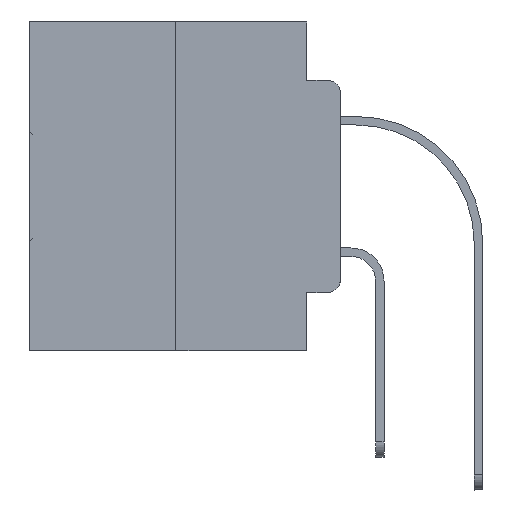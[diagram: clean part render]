
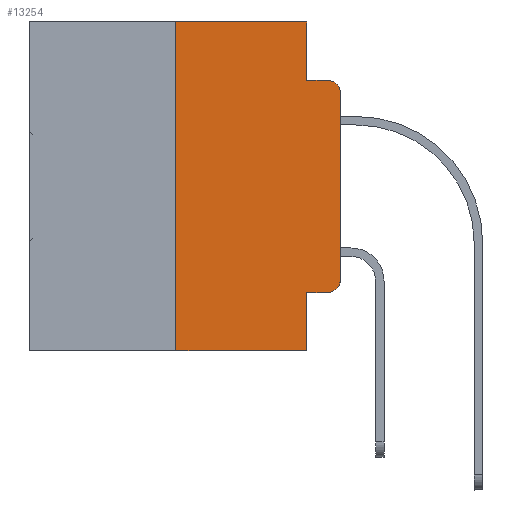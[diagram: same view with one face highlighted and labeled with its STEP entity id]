
A CAD part, left-side view. The second image highlights one B-rep face of the part: STEP entity #13254.
In plain terms, the highlighted planar face has unit normal (-1, 0, 0).
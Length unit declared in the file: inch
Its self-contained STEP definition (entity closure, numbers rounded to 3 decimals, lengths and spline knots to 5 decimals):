
#569 = VECTOR ( 'NONE', #16032, 39.37008 ) ;
#647 = DIRECTION ( 'NONE',  ( 0., -1., 0. ) ) ;
#1013 = ORIENTED_EDGE ( 'NONE', *, *, #14239, .T. ) ;
#1118 = DIRECTION ( 'NONE',  ( 0., 0., 1. ) ) ;
#1157 = DIRECTION ( 'NONE',  ( 0., 0., -1. ) ) ;
#1523 = ORIENTED_EDGE ( 'NONE', *, *, #28385, .T. ) ;
#1651 = CIRCLE ( 'NONE', #7608, 0.02 ) ;
#1792 = ORIENTED_EDGE ( 'NONE', *, *, #4485, .F. ) ;
#2020 = EDGE_CURVE ( 'NONE', #20331, #15721, #5002, .T. ) ;
#2157 = CARTESIAN_POINT ( 'NONE',  ( 0., 0.473, 0. ) ) ;
#2500 = VERTEX_POINT ( 'NONE', #3245 ) ;
#2501 = EDGE_LOOP ( 'NONE', ( #1523, #11395, #4385, #7156, #28050, #1792, #4592, #26779, #1013, #17779 ) ) ;
#2901 = VERTEX_POINT ( 'NONE', #24374 ) ;
#3165 = EDGE_CURVE ( 'NONE', #2500, #25275, #1651, .T. ) ;
#3245 = CARTESIAN_POINT ( 'NONE',  ( 0., 0., -0.1085 ) ) ;
#4208 = FACE_OUTER_BOUND ( 'NONE', #2501, .T. ) ;
#4333 = EDGE_CURVE ( 'NONE', #11425, #25275, #31983, .T. ) ;
#4385 = ORIENTED_EDGE ( 'NONE', *, *, #4333, .F. ) ;
#4485 = EDGE_CURVE ( 'NONE', #24267, #2901, #19437, .T. ) ;
#4533 = DIRECTION ( 'NONE',  ( -1., 0., 0. ) ) ;
#4592 = ORIENTED_EDGE ( 'NONE', *, *, #19235, .T. ) ;
#5002 = LINE ( 'NONE', #15340, #5952 ) ;
#5378 = CARTESIAN_POINT ( 'NONE',  ( 0., 0., -0.3915 ) ) ;
#5712 = LINE ( 'NONE', #31620, #569 ) ;
#5952 = VECTOR ( 'NONE', #25667, 39.37008 ) ;
#6264 = CARTESIAN_POINT ( 'NONE',  ( 0., 0.25, -0.5 ) ) ;
#6604 = AXIS2_PLACEMENT_3D ( 'NONE', #10593, #23294, #15172 ) ;
#6841 = VERTEX_POINT ( 'NONE', #17994 ) ;
#6898 = DIRECTION ( 'NONE',  ( 0., 0., -1. ) ) ;
#7156 = ORIENTED_EDGE ( 'NONE', *, *, #7508, .F. ) ;
#7508 = EDGE_CURVE ( 'NONE', #6841, #11425, #21168, .T. ) ;
#7608 = AXIS2_PLACEMENT_3D ( 'NONE', #19430, #4533, #6898 ) ;
#9150 = VERTEX_POINT ( 'NONE', #5378 ) ;
#9640 = DIRECTION ( 'NONE',  ( 0., 0., -1. ) ) ;
#9806 = PLANE ( 'NONE',  #13371 ) ;
#10593 = CARTESIAN_POINT ( 'NONE',  ( 0., 0.02, -0.3915 ) ) ;
#11395 = ORIENTED_EDGE ( 'NONE', *, *, #3165, .T. ) ;
#11425 = VERTEX_POINT ( 'NONE', #17455 ) ;
#11766 = LINE ( 'NONE', #22102, #21920 ) ;
#12451 = VECTOR ( 'NONE', #1118, 39.37008 ) ;
#12550 = CIRCLE ( 'NONE', #6604, 0.02 ) ;
#12561 = EDGE_CURVE ( 'NONE', #27626, #9150, #12550, .T. ) ;
#13227 = CARTESIAN_POINT ( 'NONE',  ( 0., 0.051, -0.5 ) ) ;
#13254 = ADVANCED_FACE ( 'NONE', ( #4208 ), #9806, .F. ) ;
#13371 = AXIS2_PLACEMENT_3D ( 'NONE', #2157, #29968, #9640 ) ;
#14180 = VECTOR ( 'NONE', #30111, 39.37008 ) ;
#14239 = EDGE_CURVE ( 'NONE', #20331, #27626, #17836, .T. ) ;
#14314 = CARTESIAN_POINT ( 'NONE',  ( 0., 0.02, -0.0885 ) ) ;
#15172 = DIRECTION ( 'NONE',  ( 0., 0., -1. ) ) ;
#15340 = CARTESIAN_POINT ( 'NONE',  ( 0., 0.051, 0. ) ) ;
#15721 = VERTEX_POINT ( 'NONE', #13227 ) ;
#16032 = DIRECTION ( 'NONE',  ( 0., -1., 0. ) ) ;
#17455 = CARTESIAN_POINT ( 'NONE',  ( 0., 0.051, -0.0885 ) ) ;
#17779 = ORIENTED_EDGE ( 'NONE', *, *, #12561, .T. ) ;
#17836 = LINE ( 'NONE', #20875, #28039 ) ;
#17994 = CARTESIAN_POINT ( 'NONE',  ( 0., 0.051, 0. ) ) ;
#19235 = EDGE_CURVE ( 'NONE', #24267, #15721, #5712, .T. ) ;
#19430 = CARTESIAN_POINT ( 'NONE',  ( 0., 0.02, -0.1085 ) ) ;
#19437 = LINE ( 'NONE', #19611, #14180 ) ;
#19611 = CARTESIAN_POINT ( 'NONE',  ( 0., 0.25, 0. ) ) ;
#20331 = VERTEX_POINT ( 'NONE', #31530 ) ;
#20875 = CARTESIAN_POINT ( 'NONE',  ( 0., 0.051, -0.4115 ) ) ;
#21168 = LINE ( 'NONE', #21496, #30901 ) ;
#21496 = CARTESIAN_POINT ( 'NONE',  ( 0., 0.051, 0. ) ) ;
#21920 = VECTOR ( 'NONE', #32427, 39.37008 ) ;
#22102 = CARTESIAN_POINT ( 'NONE',  ( 0., 0.473, 0. ) ) ;
#22520 = CARTESIAN_POINT ( 'NONE',  ( 0., 0.02, -0.4115 ) ) ;
#23092 = DIRECTION ( 'NONE',  ( 0., -1., 0. ) ) ;
#23294 = DIRECTION ( 'NONE',  ( -1., 0., 0. ) ) ;
#23367 = VECTOR ( 'NONE', #647, 39.37008 ) ;
#23872 = CARTESIAN_POINT ( 'NONE',  ( 0., 0.051, -0.0885 ) ) ;
#24267 = VERTEX_POINT ( 'NONE', #6264 ) ;
#24374 = CARTESIAN_POINT ( 'NONE',  ( 0., 0.25, 0. ) ) ;
#25014 = CARTESIAN_POINT ( 'NONE',  ( 0., 0., 0. ) ) ;
#25275 = VERTEX_POINT ( 'NONE', #14314 ) ;
#25667 = DIRECTION ( 'NONE',  ( 0., 0., -1. ) ) ;
#26779 = ORIENTED_EDGE ( 'NONE', *, *, #2020, .F. ) ;
#27626 = VERTEX_POINT ( 'NONE', #22520 ) ;
#28039 = VECTOR ( 'NONE', #23092, 39.37008 ) ;
#28050 = ORIENTED_EDGE ( 'NONE', *, *, #31520, .F. ) ;
#28385 = EDGE_CURVE ( 'NONE', #9150, #2500, #29750, .T. ) ;
#29750 = LINE ( 'NONE', #25014, #12451 ) ;
#29968 = DIRECTION ( 'NONE',  ( 1., 0., 0. ) ) ;
#30111 = DIRECTION ( 'NONE',  ( 0., 0., 1. ) ) ;
#30901 = VECTOR ( 'NONE', #1157, 39.37008 ) ;
#31520 = EDGE_CURVE ( 'NONE', #2901, #6841, #11766, .T. ) ;
#31530 = CARTESIAN_POINT ( 'NONE',  ( 0., 0.051, -0.4115 ) ) ;
#31620 = CARTESIAN_POINT ( 'NONE',  ( 0., 0.473, -0.5 ) ) ;
#31983 = LINE ( 'NONE', #23872, #23367 ) ;
#32427 = DIRECTION ( 'NONE',  ( 0., -1., 0. ) ) ;
